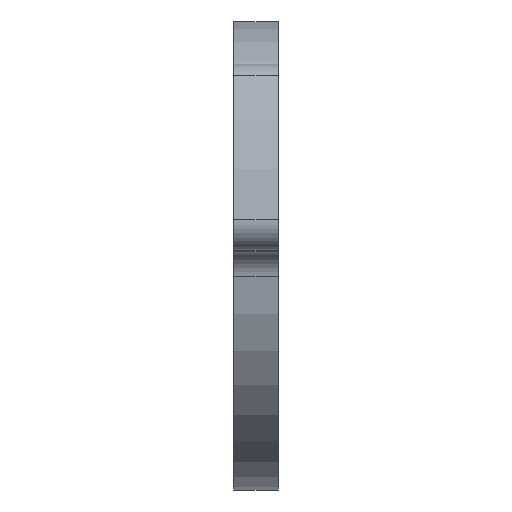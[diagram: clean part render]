
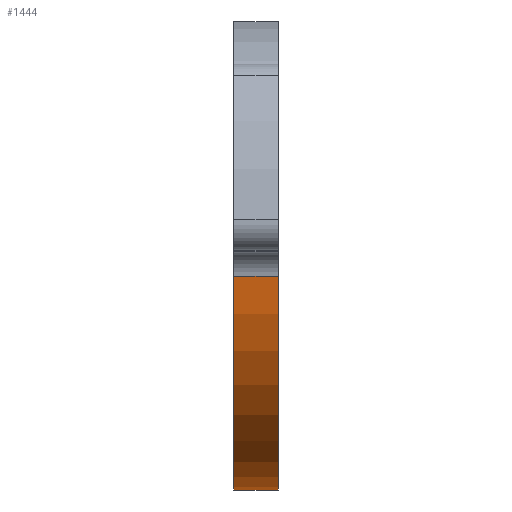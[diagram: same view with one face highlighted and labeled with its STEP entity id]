
A CAD part, front view. The second image highlights one B-rep face of the part: STEP entity #1444.
In plain terms, the highlighted cylindrical face has radius 17 mm (diameter 34 mm), a partial arc.
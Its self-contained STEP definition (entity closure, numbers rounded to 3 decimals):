
#44 = PLANE('',#45);
#45 = AXIS2_PLACEMENT_3D('',#46,#47,#48);
#46 = CARTESIAN_POINT('',(133.2,-0.049,-0.218));
#47 = DIRECTION('',(1.,0.,0.));
#48 = DIRECTION('',(0.,0.,1.));
#72 = CYLINDRICAL_SURFACE('',#73,2.);
#73 = AXIS2_PLACEMENT_3D('',#74,#75,#76);
#74 = CARTESIAN_POINT('',(130.,-18.926,-1.67));
#75 = DIRECTION('',(1.,0.,0.));
#76 = DIRECTION('',(0.,0.017,
    1.));
#100 = PLANE('',#101);
#101 = AXIS2_PLACEMENT_3D('',#102,#103,#104);
#102 = CARTESIAN_POINT('',(130.,-0.049,-0.218));
#103 = DIRECTION('',(-1.,-0.,-0.));
#104 = DIRECTION('',(0.,0.,-1.));
#499 = VERTEX_POINT('',#500);
#500 = CARTESIAN_POINT('',(133.2,-16.934,-1.494));
#526 = EDGE_CURVE('',#499,#527,#529,.T.);
#527 = VERTEX_POINT('',#528);
#528 = CARTESIAN_POINT('',(133.2,0.,-17.));
#529 = SURFACE_CURVE('',#530,(#535,#542),.PCURVE_S1.);
#530 = CIRCLE('',#531,17.);
#531 = AXIS2_PLACEMENT_3D('',#532,#533,#534);
#532 = CARTESIAN_POINT('',(133.2,0.,0.));
#533 = DIRECTION('',(1.,-0.,0.));
#534 = DIRECTION('',(0.,0.,-1.));
#535 = PCURVE('',#44,#536);
#536 = DEFINITIONAL_REPRESENTATION('',(#537),#541);
#537 = CIRCLE('',#538,17.);
#538 = AXIS2_PLACEMENT_2D('',#539,#540);
#539 = CARTESIAN_POINT('',(0.218,-0.049));
#540 = DIRECTION('',(-1.,0.));
#541 = ( GEOMETRIC_REPRESENTATION_CONTEXT(2) 
PARAMETRIC_REPRESENTATION_CONTEXT() REPRESENTATION_CONTEXT('2D SPACE',''
  ) );
#542 = PCURVE('',#543,#548);
#543 = CYLINDRICAL_SURFACE('',#544,17.);
#544 = AXIS2_PLACEMENT_3D('',#545,#546,#547);
#545 = CARTESIAN_POINT('',(130.,0.,0.));
#546 = DIRECTION('',(1.,0.,0.));
#547 = DIRECTION('',(0.,0.,-1.));
#548 = DEFINITIONAL_REPRESENTATION('',(#549),#553);
#549 = LINE('',#550,#551);
#550 = CARTESIAN_POINT('',(0.,3.2));
#551 = VECTOR('',#552,1.);
#552 = DIRECTION('',(1.,0.));
#553 = ( GEOMETRIC_REPRESENTATION_CONTEXT(2) 
PARAMETRIC_REPRESENTATION_CONTEXT() REPRESENTATION_CONTEXT('2D SPACE',''
  ) );
#555 = EDGE_CURVE('',#527,#556,#558,.T.);
#556 = VERTEX_POINT('',#557);
#557 = CARTESIAN_POINT('',(133.2,11.8,-12.237));
#558 = SURFACE_CURVE('',#559,(#564,#571),.PCURVE_S1.);
#559 = CIRCLE('',#560,17.);
#560 = AXIS2_PLACEMENT_3D('',#561,#562,#563);
#561 = CARTESIAN_POINT('',(133.2,0.,0.));
#562 = DIRECTION('',(1.,-0.,0.));
#563 = DIRECTION('',(0.,0.,-1.));
#564 = PCURVE('',#44,#565);
#565 = DEFINITIONAL_REPRESENTATION('',(#566),#570);
#566 = CIRCLE('',#567,17.);
#567 = AXIS2_PLACEMENT_2D('',#568,#569);
#568 = CARTESIAN_POINT('',(0.218,-0.049));
#569 = DIRECTION('',(-1.,0.));
#570 = ( GEOMETRIC_REPRESENTATION_CONTEXT(2) 
PARAMETRIC_REPRESENTATION_CONTEXT() REPRESENTATION_CONTEXT('2D SPACE',''
  ) );
#571 = PCURVE('',#543,#572);
#572 = DEFINITIONAL_REPRESENTATION('',(#573),#577);
#573 = LINE('',#574,#575);
#574 = CARTESIAN_POINT('',(6.283,3.2));
#575 = VECTOR('',#576,1.);
#576 = DIRECTION('',(1.,0.));
#577 = ( GEOMETRIC_REPRESENTATION_CONTEXT(2) 
PARAMETRIC_REPRESENTATION_CONTEXT() REPRESENTATION_CONTEXT('2D SPACE',''
  ) );
#598 = CYLINDRICAL_SURFACE('',#599,2.);
#599 = AXIS2_PLACEMENT_3D('',#600,#601,#602);
#600 = CARTESIAN_POINT('',(130.,13.188,-13.677));
#601 = DIRECTION('',(1.,0.,0.));
#602 = DIRECTION('',(0.,-0.694,0.72)
  );
#741 = VERTEX_POINT('',#742);
#742 = CARTESIAN_POINT('',(130.,-16.934,-1.494));
#764 = EDGE_CURVE('',#741,#499,#765,.T.);
#765 = SURFACE_CURVE('',#766,(#770,#777),.PCURVE_S1.);
#766 = LINE('',#767,#768);
#767 = CARTESIAN_POINT('',(130.,-16.934,-1.494));
#768 = VECTOR('',#769,1.);
#769 = DIRECTION('',(1.,0.,0.));
#770 = PCURVE('',#72,#771);
#771 = DEFINITIONAL_REPRESENTATION('',(#772),#776);
#772 = LINE('',#773,#774);
#773 = CARTESIAN_POINT('',(-1.465,0.));
#774 = VECTOR('',#775,1.);
#775 = DIRECTION('',(-0.,1.));
#776 = ( GEOMETRIC_REPRESENTATION_CONTEXT(2) 
PARAMETRIC_REPRESENTATION_CONTEXT() REPRESENTATION_CONTEXT('2D SPACE',''
  ) );
#777 = PCURVE('',#543,#778);
#778 = DEFINITIONAL_REPRESENTATION('',(#779),#783);
#779 = LINE('',#780,#781);
#780 = CARTESIAN_POINT('',(4.8,0.));
#781 = VECTOR('',#782,1.);
#782 = DIRECTION('',(0.,1.));
#783 = ( GEOMETRIC_REPRESENTATION_CONTEXT(2) 
PARAMETRIC_REPRESENTATION_CONTEXT() REPRESENTATION_CONTEXT('2D SPACE',''
  ) );
#1124 = VERTEX_POINT('',#1125);
#1125 = CARTESIAN_POINT('',(130.,11.8,-12.237));
#1147 = EDGE_CURVE('',#1148,#1124,#1150,.T.);
#1148 = VERTEX_POINT('',#1149);
#1149 = CARTESIAN_POINT('',(130.,0.,-17.));
#1150 = SURFACE_CURVE('',#1151,(#1156,#1167),.PCURVE_S1.);
#1151 = CIRCLE('',#1152,17.);
#1152 = AXIS2_PLACEMENT_3D('',#1153,#1154,#1155);
#1153 = CARTESIAN_POINT('',(130.,0.,0.));
#1154 = DIRECTION('',(1.,-0.,0.));
#1155 = DIRECTION('',(0.,0.,-1.));
#1156 = PCURVE('',#100,#1157);
#1157 = DEFINITIONAL_REPRESENTATION('',(#1158),#1166);
#1158 = ( BOUNDED_CURVE() B_SPLINE_CURVE(2,(#1159,#1160,#1161,#1162,
#1163,#1164,#1165),.UNSPECIFIED.,.T.,.F.) B_SPLINE_CURVE_WITH_KNOTS((1,2
    ,2,2,2,1),(-2.094,0.,2.094,4.189,
6.283,8.378),.UNSPECIFIED.) CURVE() 
GEOMETRIC_REPRESENTATION_ITEM() RATIONAL_B_SPLINE_CURVE((1.,0.5,1.,0.5,
1.,0.5,1.)) REPRESENTATION_ITEM('') );
#1159 = CARTESIAN_POINT('',(16.782,-0.049));
#1160 = CARTESIAN_POINT('',(16.782,-29.493));
#1161 = CARTESIAN_POINT('',(-8.718,-14.771));
#1162 = CARTESIAN_POINT('',(-34.218,-0.049));
#1163 = CARTESIAN_POINT('',(-8.718,14.674));
#1164 = CARTESIAN_POINT('',(16.782,29.396));
#1165 = CARTESIAN_POINT('',(16.782,-0.049));
#1166 = ( GEOMETRIC_REPRESENTATION_CONTEXT(2) 
PARAMETRIC_REPRESENTATION_CONTEXT() REPRESENTATION_CONTEXT('2D SPACE',''
  ) );
#1167 = PCURVE('',#543,#1168);
#1168 = DEFINITIONAL_REPRESENTATION('',(#1169),#1173);
#1169 = LINE('',#1170,#1171);
#1170 = CARTESIAN_POINT('',(6.283,0.));
#1171 = VECTOR('',#1172,1.);
#1172 = DIRECTION('',(1.,0.));
#1173 = ( GEOMETRIC_REPRESENTATION_CONTEXT(2) 
PARAMETRIC_REPRESENTATION_CONTEXT() REPRESENTATION_CONTEXT('2D SPACE',''
  ) );
#1175 = EDGE_CURVE('',#741,#1148,#1176,.T.);
#1176 = SURFACE_CURVE('',#1177,(#1182,#1193),.PCURVE_S1.);
#1177 = CIRCLE('',#1178,17.);
#1178 = AXIS2_PLACEMENT_3D('',#1179,#1180,#1181);
#1179 = CARTESIAN_POINT('',(130.,0.,0.));
#1180 = DIRECTION('',(1.,-0.,0.));
#1181 = DIRECTION('',(0.,0.,-1.));
#1182 = PCURVE('',#100,#1183);
#1183 = DEFINITIONAL_REPRESENTATION('',(#1184),#1192);
#1184 = ( BOUNDED_CURVE() B_SPLINE_CURVE(2,(#1185,#1186,#1187,#1188,
#1189,#1190,#1191),.UNSPECIFIED.,.T.,.F.) B_SPLINE_CURVE_WITH_KNOTS((1,2
    ,2,2,2,1),(-2.094,0.,2.094,4.189,
6.283,8.378),.UNSPECIFIED.) CURVE() 
GEOMETRIC_REPRESENTATION_ITEM() RATIONAL_B_SPLINE_CURVE((1.,0.5,1.,0.5,
1.,0.5,1.)) REPRESENTATION_ITEM('') );
#1185 = CARTESIAN_POINT('',(16.782,-0.049));
#1186 = CARTESIAN_POINT('',(16.782,-29.493));
#1187 = CARTESIAN_POINT('',(-8.718,-14.771));
#1188 = CARTESIAN_POINT('',(-34.218,-0.049));
#1189 = CARTESIAN_POINT('',(-8.718,14.674));
#1190 = CARTESIAN_POINT('',(16.782,29.396));
#1191 = CARTESIAN_POINT('',(16.782,-0.049));
#1192 = ( GEOMETRIC_REPRESENTATION_CONTEXT(2) 
PARAMETRIC_REPRESENTATION_CONTEXT() REPRESENTATION_CONTEXT('2D SPACE',''
  ) );
#1193 = PCURVE('',#543,#1194);
#1194 = DEFINITIONAL_REPRESENTATION('',(#1195),#1199);
#1195 = LINE('',#1196,#1197);
#1196 = CARTESIAN_POINT('',(0.,0.));
#1197 = VECTOR('',#1198,1.);
#1198 = DIRECTION('',(1.,0.));
#1199 = ( GEOMETRIC_REPRESENTATION_CONTEXT(2) 
PARAMETRIC_REPRESENTATION_CONTEXT() REPRESENTATION_CONTEXT('2D SPACE',''
  ) );
#1397 = EDGE_CURVE('',#1124,#556,#1398,.T.);
#1398 = SURFACE_CURVE('',#1399,(#1403,#1410),.PCURVE_S1.);
#1399 = LINE('',#1400,#1401);
#1400 = CARTESIAN_POINT('',(130.,11.8,-12.237));
#1401 = VECTOR('',#1402,1.);
#1402 = DIRECTION('',(1.,0.,0.));
#1403 = PCURVE('',#598,#1404);
#1404 = DEFINITIONAL_REPRESENTATION('',(#1405),#1409);
#1405 = LINE('',#1406,#1407);
#1406 = CARTESIAN_POINT('',(-0.,0.));
#1407 = VECTOR('',#1408,1.);
#1408 = DIRECTION('',(-0.,1.));
#1409 = ( GEOMETRIC_REPRESENTATION_CONTEXT(2) 
PARAMETRIC_REPRESENTATION_CONTEXT() REPRESENTATION_CONTEXT('2D SPACE',''
  ) );
#1410 = PCURVE('',#543,#1411);
#1411 = DEFINITIONAL_REPRESENTATION('',(#1412),#1416);
#1412 = LINE('',#1413,#1414);
#1413 = CARTESIAN_POINT('',(7.05,0.));
#1414 = VECTOR('',#1415,1.);
#1415 = DIRECTION('',(0.,1.));
#1416 = ( GEOMETRIC_REPRESENTATION_CONTEXT(2) 
PARAMETRIC_REPRESENTATION_CONTEXT() REPRESENTATION_CONTEXT('2D SPACE',''
  ) );
#1444 = ADVANCED_FACE('',(#1445),#543,.T.);
#1445 = FACE_BOUND('',#1446,.T.);
#1446 = EDGE_LOOP('',(#1447,#1448,#1449,#1450,#1451,#1452));
#1447 = ORIENTED_EDGE('',*,*,#1147,.T.);
#1448 = ORIENTED_EDGE('',*,*,#1397,.T.);
#1449 = ORIENTED_EDGE('',*,*,#555,.F.);
#1450 = ORIENTED_EDGE('',*,*,#526,.F.);
#1451 = ORIENTED_EDGE('',*,*,#764,.F.);
#1452 = ORIENTED_EDGE('',*,*,#1175,.T.);
